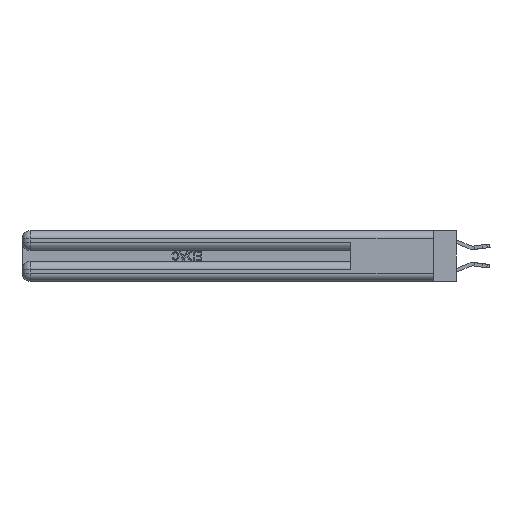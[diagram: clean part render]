
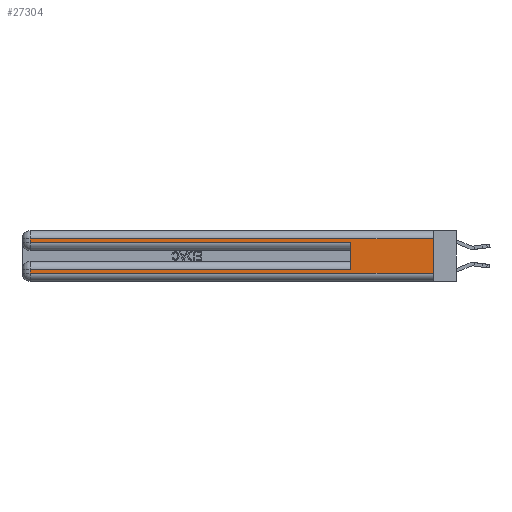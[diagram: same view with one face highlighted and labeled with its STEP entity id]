
A CAD part, left-side view. The second image highlights one B-rep face of the part: STEP entity #27304.
In plain terms, the highlighted planar face has unit normal (-1, 0, 0).
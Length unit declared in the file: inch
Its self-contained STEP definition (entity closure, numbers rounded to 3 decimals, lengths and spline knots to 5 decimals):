
#106 = ORIENTED_EDGE ( 'NONE', *, *, #10735, .T. ) ;
#263 = CARTESIAN_POINT ( 'NONE',  ( 0., 0.6, 0.085 ) ) ;
#844 = VECTOR ( 'NONE', #28869, 39.37008 ) ;
#1250 = EDGE_CURVE ( 'NONE', #24446, #1504, #23414, .T. ) ;
#1504 = VERTEX_POINT ( 'NONE', #20898 ) ;
#2361 = DIRECTION ( 'NONE',  ( 0., 0., -1. ) ) ;
#2494 = VECTOR ( 'NONE', #13592, 39.37008 ) ;
#2947 = ORIENTED_EDGE ( 'NONE', *, *, #25511, .T. ) ;
#3043 = AXIS2_PLACEMENT_3D ( 'NONE', #13735, #16025, #2361 ) ;
#3325 = EDGE_LOOP ( 'NONE', ( #10054, #23591, #23932, #29365, #22023, #27068, #2947, #106 ) ) ;
#3511 = LINE ( 'NONE', #19162, #8897 ) ;
#4360 = CARTESIAN_POINT ( 'NONE',  ( 0., 2.94, 0.085 ) ) ;
#5022 = CARTESIAN_POINT ( 'NONE',  ( 0., 2.94, 0.31 ) ) ;
#5885 = VECTOR ( 'NONE', #11135, 39.37008 ) ;
#6824 = EDGE_CURVE ( 'NONE', #14391, #13618, #12957, .T. ) ;
#6897 = CARTESIAN_POINT ( 'NONE',  ( 0., 0., 0.31 ) ) ;
#7063 = VECTOR ( 'NONE', #24069, 39.37008 ) ;
#8897 = VECTOR ( 'NONE', #23589, 39.37008 ) ;
#10054 = ORIENTED_EDGE ( 'NONE', *, *, #26342, .F. ) ;
#10381 = LINE ( 'NONE', #13469, #27757 ) ;
#10520 = CARTESIAN_POINT ( 'NONE',  ( 0., 0., 0.06 ) ) ;
#10735 = EDGE_CURVE ( 'NONE', #11598, #14477, #13140, .T. ) ;
#10792 = EDGE_CURVE ( 'NONE', #19588, #24446, #20780, .T. ) ;
#11135 = DIRECTION ( 'NONE',  ( 0., 0., 1. ) ) ;
#11598 = VERTEX_POINT ( 'NONE', #15346 ) ;
#11981 = LINE ( 'NONE', #15597, #5885 ) ;
#12027 = CARTESIAN_POINT ( 'NONE',  ( 0., 0., 0.06 ) ) ;
#12957 = LINE ( 'NONE', #19732, #844 ) ;
#13127 = EDGE_CURVE ( 'NONE', #1504, #24654, #26695, .T. ) ;
#13140 = LINE ( 'NONE', #10520, #7063 ) ;
#13305 = DIRECTION ( 'NONE',  ( 0., 0., -1. ) ) ;
#13469 = CARTESIAN_POINT ( 'NONE',  ( 0., 2.94, 0.37 ) ) ;
#13592 = DIRECTION ( 'NONE',  ( 0., -1., 0. ) ) ;
#13618 = VERTEX_POINT ( 'NONE', #4360 ) ;
#13735 = CARTESIAN_POINT ( 'NONE',  ( 0., 0., 0.37 ) ) ;
#14391 = VERTEX_POINT ( 'NONE', #263 ) ;
#14477 = VERTEX_POINT ( 'NONE', #12027 ) ;
#15188 = DIRECTION ( 'NONE',  ( 0., 1., 0. ) ) ;
#15346 = CARTESIAN_POINT ( 'NONE',  ( 0., 2.94, 0.06 ) ) ;
#15597 = CARTESIAN_POINT ( 'NONE',  ( 0., 0.6, 0.145 ) ) ;
#15755 = DIRECTION ( 'NONE',  ( 0., 0., -1. ) ) ;
#16025 = DIRECTION ( 'NONE',  ( 1., 0., 0. ) ) ;
#16709 = FACE_OUTER_BOUND ( 'NONE', #3325, .T. ) ;
#17419 = VECTOR ( 'NONE', #13305, 39.37008 ) ;
#19162 = CARTESIAN_POINT ( 'NONE',  ( 0., 0., 0.37 ) ) ;
#19434 = EDGE_CURVE ( 'NONE', #14391, #24654, #11981, .T. ) ;
#19588 = VERTEX_POINT ( 'NONE', #6897 ) ;
#19732 = CARTESIAN_POINT ( 'NONE',  ( 0., 0., 0.085 ) ) ;
#20085 = VECTOR ( 'NONE', #15188, 39.37008 ) ;
#20780 = LINE ( 'NONE', #26490, #20085 ) ;
#20898 = CARTESIAN_POINT ( 'NONE',  ( 0., 2.94, 0.285 ) ) ;
#22023 = ORIENTED_EDGE ( 'NONE', *, *, #19434, .F. ) ;
#23414 = LINE ( 'NONE', #24481, #17419 ) ;
#23589 = DIRECTION ( 'NONE',  ( 0., 0., -1. ) ) ;
#23591 = ORIENTED_EDGE ( 'NONE', *, *, #10792, .T. ) ;
#23932 = ORIENTED_EDGE ( 'NONE', *, *, #1250, .T. ) ;
#24069 = DIRECTION ( 'NONE',  ( 0., -1., 0. ) ) ;
#24187 = CARTESIAN_POINT ( 'NONE',  ( 0., 0.6, 0.285 ) ) ;
#24446 = VERTEX_POINT ( 'NONE', #5022 ) ;
#24481 = CARTESIAN_POINT ( 'NONE',  ( 0., 2.94, 0.37 ) ) ;
#24654 = VERTEX_POINT ( 'NONE', #24187 ) ;
#24871 = CARTESIAN_POINT ( 'NONE',  ( 0., 0., 0.285 ) ) ;
#25511 = EDGE_CURVE ( 'NONE', #13618, #11598, #10381, .T. ) ;
#26342 = EDGE_CURVE ( 'NONE', #19588, #14477, #3511, .T. ) ;
#26490 = CARTESIAN_POINT ( 'NONE',  ( 0., 0., 0.31 ) ) ;
#26695 = LINE ( 'NONE', #24871, #2494 ) ;
#27068 = ORIENTED_EDGE ( 'NONE', *, *, #6824, .T. ) ;
#27304 = ADVANCED_FACE ( 'NONE', ( #16709 ), #27320, .F. ) ;
#27320 = PLANE ( 'NONE',  #3043 ) ;
#27757 = VECTOR ( 'NONE', #15755, 39.37008 ) ;
#28869 = DIRECTION ( 'NONE',  ( 0., 1., 0. ) ) ;
#29365 = ORIENTED_EDGE ( 'NONE', *, *, #13127, .T. ) ;
